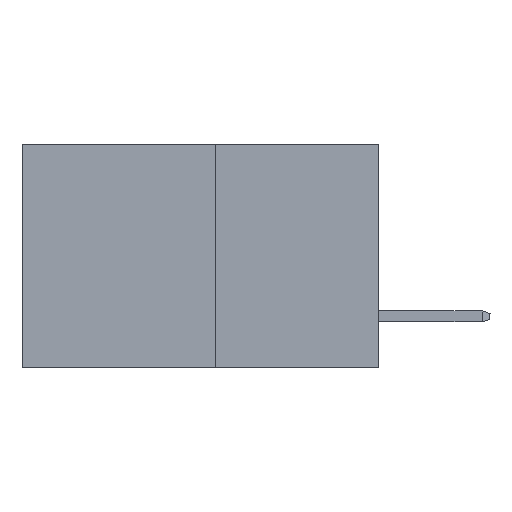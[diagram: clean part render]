
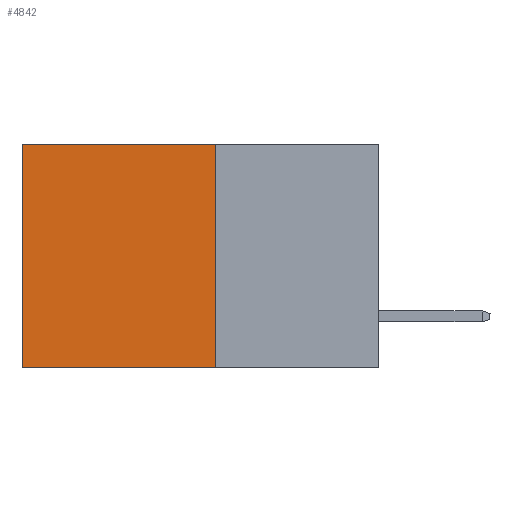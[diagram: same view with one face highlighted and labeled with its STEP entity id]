
A CAD part, left-side view. The second image highlights one B-rep face of the part: STEP entity #4842.
In plain terms, the highlighted planar face has unit normal (-1, 0, 0).
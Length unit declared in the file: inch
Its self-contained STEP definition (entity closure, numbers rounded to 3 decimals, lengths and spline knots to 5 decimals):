
#419 = ORIENTED_EDGE ( 'NONE', *, *, #9555, .F. ) ;
#591 = ORIENTED_EDGE ( 'NONE', *, *, #9953, .T. ) ;
#1140 = LINE ( 'NONE', #5989, #7901 ) ;
#1222 = CARTESIAN_POINT ( 'NONE',  ( 0.277, 0.27, 0. ) ) ;
#1572 = VECTOR ( 'NONE', #10519, 39.37008 ) ;
#1586 = CARTESIAN_POINT ( 'NONE',  ( 0.277, 0.27, -0.37 ) ) ;
#2391 = EDGE_LOOP ( 'NONE', ( #591, #419, #8084, #3820 ) ) ;
#2627 = FACE_OUTER_BOUND ( 'NONE', #2391, .T. ) ;
#2740 = CARTESIAN_POINT ( 'NONE',  ( 0.277, 0.59, -0.37 ) ) ;
#3350 = DIRECTION ( 'NONE',  ( 0., 0., -1. ) ) ;
#3383 = DIRECTION ( 'NONE',  ( 0., 0., -1. ) ) ;
#3506 = AXIS2_PLACEMENT_3D ( 'NONE', #1586, #8636, #3350 ) ;
#3820 = ORIENTED_EDGE ( 'NONE', *, *, #4557, .T. ) ;
#3998 = CARTESIAN_POINT ( 'NONE',  ( 0.277, 0.59, 0. ) ) ;
#4511 = VERTEX_POINT ( 'NONE', #10710 ) ;
#4557 = EDGE_CURVE ( 'NONE', #8619, #6486, #10222, .T. ) ;
#4809 = CARTESIAN_POINT ( 'NONE',  ( 0.277, 0.27, -0.37 ) ) ;
#4842 = ADVANCED_FACE ( 'NONE', ( #2627 ), #7716, .F. ) ;
#5572 = DIRECTION ( 'NONE',  ( 0., 1., 0. ) ) ;
#5603 = VECTOR ( 'NONE', #5572, 39.37008 ) ;
#5638 = CARTESIAN_POINT ( 'NONE',  ( 0.277, 0.59, -0.37 ) ) ;
#5648 = VECTOR ( 'NONE', #8357, 39.37008 ) ;
#5989 = CARTESIAN_POINT ( 'NONE',  ( 0.277, 0.27, -0.37 ) ) ;
#6486 = VERTEX_POINT ( 'NONE', #3998 ) ;
#7673 = CARTESIAN_POINT ( 'NONE',  ( 0.277, 0.27, 0. ) ) ;
#7716 = PLANE ( 'NONE',  #3506 ) ;
#7901 = VECTOR ( 'NONE', #3383, 39.37008 ) ;
#8048 = LINE ( 'NONE', #4809, #5648 ) ;
#8084 = ORIENTED_EDGE ( 'NONE', *, *, #9776, .F. ) ;
#8357 = DIRECTION ( 'NONE',  ( 0., 1., 0. ) ) ;
#8619 = VERTEX_POINT ( 'NONE', #7673 ) ;
#8636 = DIRECTION ( 'NONE',  ( 1., 0., 0. ) ) ;
#8876 = LINE ( 'NONE', #2740, #1572 ) ;
#9549 = VERTEX_POINT ( 'NONE', #5638 ) ;
#9555 = EDGE_CURVE ( 'NONE', #4511, #9549, #8048, .T. ) ;
#9776 = EDGE_CURVE ( 'NONE', #8619, #4511, #1140, .T. ) ;
#9953 = EDGE_CURVE ( 'NONE', #6486, #9549, #8876, .T. ) ;
#10222 = LINE ( 'NONE', #1222, #5603 ) ;
#10519 = DIRECTION ( 'NONE',  ( 0., 0., -1. ) ) ;
#10710 = CARTESIAN_POINT ( 'NONE',  ( 0.277, 0.27, -0.37 ) ) ;
